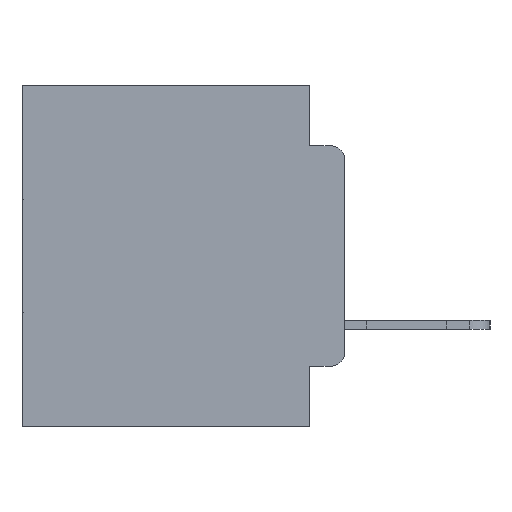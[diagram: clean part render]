
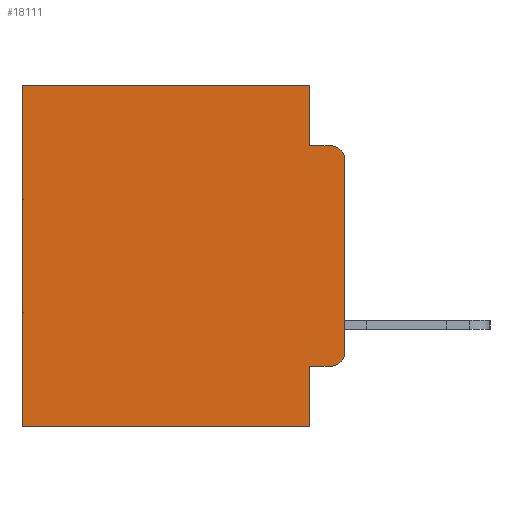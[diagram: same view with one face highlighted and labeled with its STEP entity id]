
A CAD part, left-side view. The second image highlights one B-rep face of the part: STEP entity #18111.
In plain terms, the highlighted planar face has unit normal (-1, 0, 0).
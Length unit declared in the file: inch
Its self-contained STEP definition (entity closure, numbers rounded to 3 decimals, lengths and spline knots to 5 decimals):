
#1263 = FACE_OUTER_BOUND ( 'NONE', #9913, .T. ) ;
#2139 = EDGE_CURVE ( 'NONE', #19318, #18479, #28939, .T. ) ;
#2841 = LINE ( 'NONE', #11341, #15029 ) ;
#2974 = CARTESIAN_POINT ( 'NONE',  ( 0.298, 0.02, -0.3915 ) ) ;
#3379 = VECTOR ( 'NONE', #16580, 39.37008 ) ;
#4096 = LINE ( 'NONE', #24734, #25481 ) ;
#4232 = VERTEX_POINT ( 'NONE', #8201 ) ;
#4599 = ORIENTED_EDGE ( 'NONE', *, *, #19609, .T. ) ;
#4737 = CARTESIAN_POINT ( 'NONE',  ( 0.298, 0., -0.1085 ) ) ;
#5283 = CARTESIAN_POINT ( 'NONE',  ( 0.298, 0., -0.3915 ) ) ;
#5318 = EDGE_CURVE ( 'NONE', #21513, #16801, #18386, .T. ) ;
#5629 = DIRECTION ( 'NONE',  ( 0., 0., -1. ) ) ;
#5891 = CARTESIAN_POINT ( 'NONE',  ( 0.298, 0.02, -0.0885 ) ) ;
#6662 = AXIS2_PLACEMENT_3D ( 'NONE', #11899, #30075, #16657 ) ;
#7638 = VECTOR ( 'NONE', #10823, 39.37008 ) ;
#7883 = VERTEX_POINT ( 'NONE', #4737 ) ;
#8201 = CARTESIAN_POINT ( 'NONE',  ( 0.298, 0.02, -0.4115 ) ) ;
#8757 = CARTESIAN_POINT ( 'NONE',  ( 0.298, 0., 0. ) ) ;
#9913 = EDGE_LOOP ( 'NONE', ( #25491, #16521, #12174, #26168, #17251, #21622, #14059, #18747, #23137, #4599 ) ) ;
#10316 = CARTESIAN_POINT ( 'NONE',  ( 0.298, 0.051, -0.0885 ) ) ;
#10823 = DIRECTION ( 'NONE',  ( 0., 0., -1. ) ) ;
#11181 = VERTEX_POINT ( 'NONE', #5891 ) ;
#11341 = CARTESIAN_POINT ( 'NONE',  ( 0.298, 0.473, 0. ) ) ;
#11653 = DIRECTION ( 'NONE',  ( -1., 0., 0. ) ) ;
#11899 = CARTESIAN_POINT ( 'NONE',  ( 0.298, 0., 0. ) ) ;
#11998 = PLANE ( 'NONE',  #6662 ) ;
#12174 = ORIENTED_EDGE ( 'NONE', *, *, #18992, .F. ) ;
#12209 = VECTOR ( 'NONE', #16745, 39.37008 ) ;
#12338 = VECTOR ( 'NONE', #18945, 39.37008 ) ;
#13146 = CARTESIAN_POINT ( 'NONE',  ( 0.298, 0.051, 0. ) ) ;
#13628 = CIRCLE ( 'NONE', #17544, 0.02 ) ;
#13695 = CARTESIAN_POINT ( 'NONE',  ( 0.298, 0.051, -0.0885 ) ) ;
#13763 = DIRECTION ( 'NONE',  ( 0., 0., -1. ) ) ;
#13929 = CARTESIAN_POINT ( 'NONE',  ( 0.298, 0.051, -0.5 ) ) ;
#13978 = EDGE_CURVE ( 'NONE', #7883, #19552, #18515, .T. ) ;
#13993 = LINE ( 'NONE', #13146, #7638 ) ;
#14059 = ORIENTED_EDGE ( 'NONE', *, *, #2139, .F. ) ;
#15029 = VECTOR ( 'NONE', #13763, 39.37008 ) ;
#15528 = DIRECTION ( 'NONE',  ( 0., 0., -1. ) ) ;
#16230 = CARTESIAN_POINT ( 'NONE',  ( 0.298, 0., 0. ) ) ;
#16521 = ORIENTED_EDGE ( 'NONE', *, *, #19339, .T. ) ;
#16580 = DIRECTION ( 'NONE',  ( 0., 1., 0. ) ) ;
#16635 = CARTESIAN_POINT ( 'NONE',  ( 0.298, 0.051, 0. ) ) ;
#16657 = DIRECTION ( 'NONE',  ( 0., 0., -1. ) ) ;
#16745 = DIRECTION ( 'NONE',  ( 0., 1., 0. ) ) ;
#16781 = VERTEX_POINT ( 'NONE', #29883 ) ;
#16801 = VERTEX_POINT ( 'NONE', #21093 ) ;
#16955 = AXIS2_PLACEMENT_3D ( 'NONE', #2974, #19771, #5629 ) ;
#17170 = CIRCLE ( 'NONE', #16955, 0.02 ) ;
#17251 = ORIENTED_EDGE ( 'NONE', *, *, #5318, .T. ) ;
#17360 = DIRECTION ( 'NONE',  ( 0., -1., 0. ) ) ;
#17544 = AXIS2_PLACEMENT_3D ( 'NONE', #25473, #11653, #27631 ) ;
#17587 = VECTOR ( 'NONE', #17360, 39.37008 ) ;
#18111 = ADVANCED_FACE ( 'NONE', ( #1263 ), #11998, .F. ) ;
#18386 = LINE ( 'NONE', #16230, #12209 ) ;
#18479 = VERTEX_POINT ( 'NONE', #22745 ) ;
#18515 = LINE ( 'NONE', #8757, #12338 ) ;
#18747 = ORIENTED_EDGE ( 'NONE', *, *, #19108, .F. ) ;
#18945 = DIRECTION ( 'NONE',  ( 0., 0., -1. ) ) ;
#18992 = EDGE_CURVE ( 'NONE', #20353, #11181, #23775, .T. ) ;
#19108 = EDGE_CURVE ( 'NONE', #16781, #19318, #13993, .T. ) ;
#19113 = EDGE_CURVE ( 'NONE', #21513, #20353, #4096, .T. ) ;
#19252 = EDGE_CURVE ( 'NONE', #16801, #18479, #2841, .T. ) ;
#19318 = VERTEX_POINT ( 'NONE', #13929 ) ;
#19339 = EDGE_CURVE ( 'NONE', #7883, #11181, #13628, .T. ) ;
#19552 = VERTEX_POINT ( 'NONE', #5283 ) ;
#19609 = EDGE_CURVE ( 'NONE', #4232, #19552, #17170, .T. ) ;
#19771 = DIRECTION ( 'NONE',  ( -1., 0., 0. ) ) ;
#19773 = EDGE_CURVE ( 'NONE', #16781, #4232, #29474, .T. ) ;
#20353 = VERTEX_POINT ( 'NONE', #13695 ) ;
#20374 = CARTESIAN_POINT ( 'NONE',  ( 0.298, 0.051, -0.4115 ) ) ;
#20725 = CARTESIAN_POINT ( 'NONE',  ( 0.298, 0., -0.5 ) ) ;
#21093 = CARTESIAN_POINT ( 'NONE',  ( 0.298, 0.473, 0. ) ) ;
#21513 = VERTEX_POINT ( 'NONE', #16635 ) ;
#21622 = ORIENTED_EDGE ( 'NONE', *, *, #19252, .T. ) ;
#22713 = DIRECTION ( 'NONE',  ( 0., -1., 0. ) ) ;
#22745 = CARTESIAN_POINT ( 'NONE',  ( 0.298, 0.473, -0.5 ) ) ;
#23137 = ORIENTED_EDGE ( 'NONE', *, *, #19773, .T. ) ;
#23775 = LINE ( 'NONE', #10316, #17587 ) ;
#24734 = CARTESIAN_POINT ( 'NONE',  ( 0.298, 0.051, 0. ) ) ;
#25473 = CARTESIAN_POINT ( 'NONE',  ( 0.298, 0.02, -0.1085 ) ) ;
#25481 = VECTOR ( 'NONE', #15528, 39.37008 ) ;
#25491 = ORIENTED_EDGE ( 'NONE', *, *, #13978, .F. ) ;
#26168 = ORIENTED_EDGE ( 'NONE', *, *, #19113, .F. ) ;
#27631 = DIRECTION ( 'NONE',  ( 0., 0., -1. ) ) ;
#28800 = VECTOR ( 'NONE', #22713, 39.37008 ) ;
#28939 = LINE ( 'NONE', #20725, #3379 ) ;
#29474 = LINE ( 'NONE', #20374, #28800 ) ;
#29883 = CARTESIAN_POINT ( 'NONE',  ( 0.298, 0.051, -0.4115 ) ) ;
#30075 = DIRECTION ( 'NONE',  ( 1., 0., 0. ) ) ;
